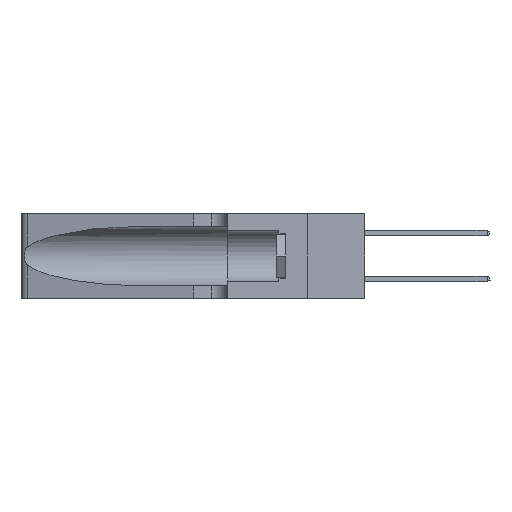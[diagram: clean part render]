
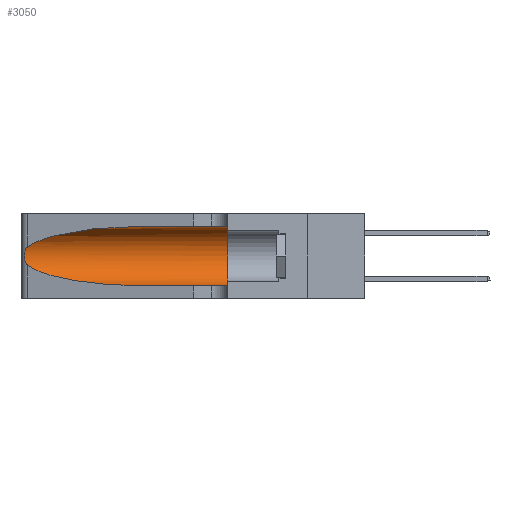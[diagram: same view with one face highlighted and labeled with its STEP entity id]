
A CAD part, left-side view. The second image highlights one B-rep face of the part: STEP entity #3050.
In plain terms, the highlighted cylindrical face has radius 3.308 mm (diameter 6.617 mm), a partial arc.
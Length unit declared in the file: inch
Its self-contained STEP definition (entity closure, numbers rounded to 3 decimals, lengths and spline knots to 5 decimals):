
#268 = CARTESIAN_POINT ( 'NONE',  ( 0.25639, 1.23184, 0.21858 ) ) ;
#314 = CARTESIAN_POINT ( 'NONE',  ( 0.25487, 1.22718, 0.22369 ) ) ;
#389 = CARTESIAN_POINT ( 'NONE',  ( 0.1305, 0.72297, 0.05475 ) ) ;
#855 = ORIENTED_EDGE ( 'NONE', *, *, #28877, .F. ) ;
#940 = VECTOR ( 'NONE', #24540, 39.37008 ) ;
#1864 = ORIENTED_EDGE ( 'NONE', *, *, #7081, .F. ) ;
#2174 = DIRECTION ( 'NONE',  ( 0., 1., 0. ) ) ;
#2513 = CARTESIAN_POINT ( 'NONE',  ( 0.1305, 0.35, 0.05475 ) ) ;
#2562 = B_SPLINE_CURVE_WITH_KNOTS ( 'NONE', 3,
 ( #3303, #10818, #268, #3183, #32310, #11061, #8502, #24622, #18893, #29623, #2941, #5615, #16437, #13738 ),
 .UNSPECIFIED., .F., .F.,
 ( 4, 2, 2, 2, 2, 2, 4 ),
 ( 0., 0.00027, 0.00053, 0.00107, 0.0016, 0.00187, 0.00214 ),
 .UNSPECIFIED. ) ;
#2770 = AXIS2_PLACEMENT_3D ( 'NONE', #18257, #20950, #13119 ) ;
#2941 = CARTESIAN_POINT ( 'NONE',  ( 0.25789, 1.23486, 0.15765 ) ) ;
#3050 = ADVANCED_FACE ( 'NONE', ( #26380 ), #10492, .F. ) ;
#3183 = CARTESIAN_POINT ( 'NONE',  ( 0.25787, 1.23484, 0.2124 ) ) ;
#3268 = VERTEX_POINT ( 'NONE', #16043 ) ;
#3303 = CARTESIAN_POINT ( 'NONE',  ( 0.25487, 1.22718, 0.22369 ) ) ;
#3354 = CARTESIAN_POINT ( 'NONE',  ( 0.18966, 0.96281, 0.31525 ) ) ;
#3969 = CARTESIAN_POINT ( 'NONE',  ( 0.18966, 0.96281, 0.05475 ) ) ;
#5343 = LINE ( 'NONE', #21945, #17009 ) ;
#5505 = EDGE_CURVE ( 'NONE', #11717, #14318, #5343, .T. ) ;
#5615 = CARTESIAN_POINT ( 'NONE',  ( 0.25639, 1.23186, 0.15144 ) ) ;
#6371 = EDGE_LOOP ( 'NONE', ( #10305, #14420, #12647, #7884, #1864, #855 ) ) ;
#7081 = EDGE_CURVE ( 'NONE', #3268, #14318, #8939, .T. ) ;
#7658 =( BOUNDED_CURVE ( )  B_SPLINE_CURVE ( 3, ( #17115, #25074, #3969, #22152 ),
 .UNSPECIFIED., .F., .T. ) 
 B_SPLINE_CURVE_WITH_KNOTS ( ( 4, 4 ),
 ( 3.44316, 4.71239 ),
 .UNSPECIFIED. ) 
 CURVE ( )  GEOMETRIC_REPRESENTATION_ITEM ( )  RATIONAL_B_SPLINE_CURVE ( ( 1., 0.87, 0.87, 1. ) ) 
 REPRESENTATION_ITEM ( '' )  );
#7884 = ORIENTED_EDGE ( 'NONE', *, *, #5505, .T. ) ;
#8502 = CARTESIAN_POINT ( 'NONE',  ( 0.26075, 1.23896, 0.19203 ) ) ;
#8939 = CIRCLE ( 'NONE', #25939, 0.13025 ) ;
#10305 = ORIENTED_EDGE ( 'NONE', *, *, #10855, .T. ) ;
#10492 = CYLINDRICAL_SURFACE ( 'NONE', #2770, 0.13025 ) ;
#10499 = EDGE_CURVE ( 'NONE', #24568, #11717, #7658, .T. ) ;
#10818 = CARTESIAN_POINT ( 'NONE',  ( 0.25555, 1.22994, 0.2215 ) ) ;
#10855 = EDGE_CURVE ( 'NONE', #11901, #14504, #30990, .T. ) ;
#11061 = CARTESIAN_POINT ( 'NONE',  ( 0.26018, 1.23835, 0.19895 ) ) ;
#11717 = VERTEX_POINT ( 'NONE', #389 ) ;
#11901 = VERTEX_POINT ( 'NONE', #26526 ) ;
#12647 = ORIENTED_EDGE ( 'NONE', *, *, #10499, .T. ) ;
#13119 = DIRECTION ( 'NONE',  ( 0., 0., -1. ) ) ;
#13738 = CARTESIAN_POINT ( 'NONE',  ( 0.25487, 1.22718, 0.14631 ) ) ;
#14259 = LINE ( 'NONE', #26746, #940 ) ;
#14318 = VERTEX_POINT ( 'NONE', #2513 ) ;
#14420 = ORIENTED_EDGE ( 'NONE', *, *, #15969, .T. ) ;
#14504 = VERTEX_POINT ( 'NONE', #21653 ) ;
#15969 = EDGE_CURVE ( 'NONE', #14504, #24568, #2562, .T. ) ;
#16043 = CARTESIAN_POINT ( 'NONE',  ( 0.1305, 0.35, 0.31525 ) ) ;
#16315 = DIRECTION ( 'NONE',  ( 0., -1., 0. ) ) ;
#16437 = CARTESIAN_POINT ( 'NONE',  ( 0.25555, 1.22993, 0.14849 ) ) ;
#17009 = VECTOR ( 'NONE', #16315, 39.37008 ) ;
#17115 = CARTESIAN_POINT ( 'NONE',  ( 0.25487, 1.22718, 0.14631 ) ) ;
#18257 = CARTESIAN_POINT ( 'NONE',  ( 0.1305, 1.61858, 0.185 ) ) ;
#18459 = CARTESIAN_POINT ( 'NONE',  ( 0.25487, 1.22718, 0.14631 ) ) ;
#18893 = CARTESIAN_POINT ( 'NONE',  ( 0.26017, 1.23833, 0.17102 ) ) ;
#20826 = DIRECTION ( 'NONE',  ( 0., 0., 1. ) ) ;
#20950 = DIRECTION ( 'NONE',  ( 0., -1., 0. ) ) ;
#21653 = CARTESIAN_POINT ( 'NONE',  ( 0.25487, 1.22718, 0.22369 ) ) ;
#21945 = CARTESIAN_POINT ( 'NONE',  ( 0.1305, 1.61858, 0.05475 ) ) ;
#22152 = CARTESIAN_POINT ( 'NONE',  ( 0.1305, 0.72297, 0.05475 ) ) ;
#24540 = DIRECTION ( 'NONE',  ( 0., -1., 0. ) ) ;
#24568 = VERTEX_POINT ( 'NONE', #18459 ) ;
#24622 = CARTESIAN_POINT ( 'NONE',  ( 0.26075, 1.23896, 0.178 ) ) ;
#25074 = CARTESIAN_POINT ( 'NONE',  ( 0.2373, 1.15595, 0.08982 ) ) ;
#25939 = AXIS2_PLACEMENT_3D ( 'NONE', #33884, #2174, #20826 ) ;
#26380 = FACE_OUTER_BOUND ( 'NONE', #6371, .T. ) ;
#26526 = CARTESIAN_POINT ( 'NONE',  ( 0.1305, 0.72297, 0.31525 ) ) ;
#26746 = CARTESIAN_POINT ( 'NONE',  ( 0.1305, 1.61858, 0.31525 ) ) ;
#27367 = CARTESIAN_POINT ( 'NONE',  ( 0.1305, 0.72297, 0.31525 ) ) ;
#28877 = EDGE_CURVE ( 'NONE', #11901, #3268, #14259, .T. ) ;
#29553 = CARTESIAN_POINT ( 'NONE',  ( 0.2373, 1.15595, 0.28018 ) ) ;
#29623 = CARTESIAN_POINT ( 'NONE',  ( 0.25856, 1.23593, 0.16098 ) ) ;
#30990 =( BOUNDED_CURVE ( )  B_SPLINE_CURVE ( 3, ( #27367, #3354, #29553, #314 ),
 .UNSPECIFIED., .F., .F. ) 
 B_SPLINE_CURVE_WITH_KNOTS ( ( 4, 4 ),
 ( 1.5708, 2.84003 ),
 .UNSPECIFIED. ) 
 CURVE ( )  GEOMETRIC_REPRESENTATION_ITEM ( )  RATIONAL_B_SPLINE_CURVE ( ( 1., 0.87, 0.87, 1. ) ) 
 REPRESENTATION_ITEM ( '' )  );
#32310 = CARTESIAN_POINT ( 'NONE',  ( 0.25854, 1.2359, 0.20912 ) ) ;
#33884 = CARTESIAN_POINT ( 'NONE',  ( 0.1305, 0.35, 0.185 ) ) ;
